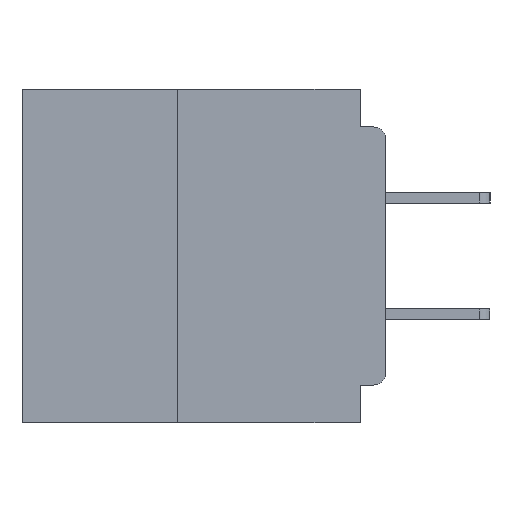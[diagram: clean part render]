
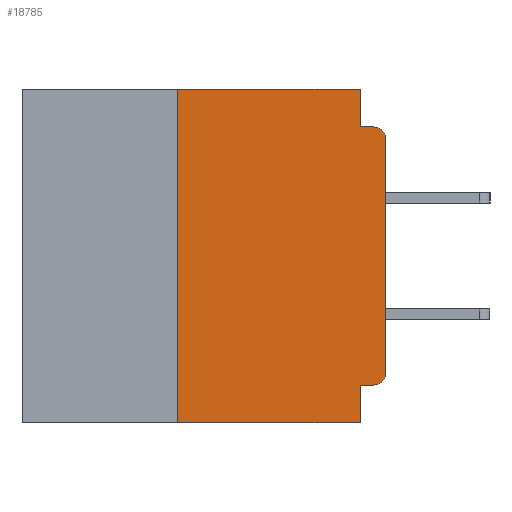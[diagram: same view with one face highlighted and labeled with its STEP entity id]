
A CAD part, left-side view. The second image highlights one B-rep face of the part: STEP entity #18785.
In plain terms, the highlighted planar face has unit normal (-1, 0, 0).
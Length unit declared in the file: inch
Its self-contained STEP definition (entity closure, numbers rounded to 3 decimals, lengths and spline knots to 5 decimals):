
#663 = CARTESIAN_POINT ( 'NONE',  ( 0., 0.015, -0.355 ) ) ;
#713 = CARTESIAN_POINT ( 'NONE',  ( 0., 0.031, -0.4 ) ) ;
#2166 = VERTEX_POINT ( 'NONE', #713 ) ;
#2674 = CARTESIAN_POINT ( 'NONE',  ( 0., 0., -0.355 ) ) ;
#2922 = VERTEX_POINT ( 'NONE', #11174 ) ;
#4207 = CARTESIAN_POINT ( 'NONE',  ( 0., 0.031, -0.045 ) ) ;
#4211 = ORIENTED_EDGE ( 'NONE', *, *, #28595, .T. ) ;
#5826 = VERTEX_POINT ( 'NONE', #27957 ) ;
#6435 = LINE ( 'NONE', #2674, #48148 ) ;
#7104 = VECTOR ( 'NONE', #25370, 39.37008 ) ;
#8493 = CARTESIAN_POINT ( 'NONE',  ( 0., 0., -0.045 ) ) ;
#8925 = AXIS2_PLACEMENT_3D ( 'NONE', #42290, #46321, #22133 ) ;
#9164 = EDGE_LOOP ( 'NONE', ( #46527, #39739, #34785, #50133, #48229, #15611, #4211, #15721, #17153, #42889 ) ) ;
#9626 = LINE ( 'NONE', #43759, #43172 ) ;
#9649 = LINE ( 'NONE', #8493, #19128 ) ;
#9907 = DIRECTION ( 'NONE',  ( 0., -1., 0. ) ) ;
#11011 = VECTOR ( 'NONE', #44878, 39.37008 ) ;
#11174 = CARTESIAN_POINT ( 'NONE',  ( 0., 0.25, 0. ) ) ;
#11696 = DIRECTION ( 'NONE',  ( -1., 0., 0. ) ) ;
#12489 = VERTEX_POINT ( 'NONE', #25854 ) ;
#12490 = CARTESIAN_POINT ( 'NONE',  ( 0., 0.25, -0.4 ) ) ;
#12646 = EDGE_CURVE ( 'NONE', #14456, #12489, #6435, .T. ) ;
#13165 = DIRECTION ( 'NONE',  ( 0., 0., -1. ) ) ;
#13948 = PLANE ( 'NONE',  #8925 ) ;
#14456 = VERTEX_POINT ( 'NONE', #663 ) ;
#15611 = ORIENTED_EDGE ( 'NONE', *, *, #50242, .F. ) ;
#15721 = ORIENTED_EDGE ( 'NONE', *, *, #23178, .F. ) ;
#16581 = VERTEX_POINT ( 'NONE', #30914 ) ;
#17153 = ORIENTED_EDGE ( 'NONE', *, *, #12646, .F. ) ;
#17453 = VERTEX_POINT ( 'NONE', #24900 ) ;
#18785 = ADVANCED_FACE ( 'NONE', ( #31189 ), #13948, .F. ) ;
#19089 = LINE ( 'NONE', #45521, #7104 ) ;
#19128 = VECTOR ( 'NONE', #28628, 39.37008 ) ;
#19195 = EDGE_CURVE ( 'NONE', #45797, #17453, #9649, .T. ) ;
#19537 = DIRECTION ( 'NONE',  ( 0., 0., -1. ) ) ;
#20698 = VERTEX_POINT ( 'NONE', #33028 ) ;
#22133 = DIRECTION ( 'NONE',  ( 0., 0., -1. ) ) ;
#22605 = CARTESIAN_POINT ( 'NONE',  ( 0., 0.015, -0.06 ) ) ;
#23178 = EDGE_CURVE ( 'NONE', #12489, #2166, #38935, .T. ) ;
#24900 = CARTESIAN_POINT ( 'NONE',  ( 0., 0.015, -0.045 ) ) ;
#25370 = DIRECTION ( 'NONE',  ( 0., 0., 1. ) ) ;
#25854 = CARTESIAN_POINT ( 'NONE',  ( 0., 0.031, -0.355 ) ) ;
#26081 = CIRCLE ( 'NONE', #33354, 0.015 ) ;
#26270 = VECTOR ( 'NONE', #9907, 39.37008 ) ;
#26529 = AXIS2_PLACEMENT_3D ( 'NONE', #35959, #11696, #40004 ) ;
#26676 = DIRECTION ( 'NONE',  ( 0., 0., -1. ) ) ;
#27008 = EDGE_CURVE ( 'NONE', #2922, #5826, #46505, .T. ) ;
#27957 = CARTESIAN_POINT ( 'NONE',  ( 0., 0.031, 0. ) ) ;
#28595 = EDGE_CURVE ( 'NONE', #20698, #2166, #45693, .T. ) ;
#28628 = DIRECTION ( 'NONE',  ( 0., -1., 0. ) ) ;
#30914 = CARTESIAN_POINT ( 'NONE',  ( 0., 0., -0.34 ) ) ;
#31189 = FACE_OUTER_BOUND ( 'NONE', #9164, .T. ) ;
#33028 = CARTESIAN_POINT ( 'NONE',  ( 0., 0.25, -0.4 ) ) ;
#33335 = EDGE_CURVE ( 'NONE', #14456, #16581, #41442, .T. ) ;
#33354 = AXIS2_PLACEMENT_3D ( 'NONE', #22605, #50775, #26676 ) ;
#33555 = CARTESIAN_POINT ( 'NONE',  ( 0., 0.031, -0.4 ) ) ;
#34110 = CARTESIAN_POINT ( 'NONE',  ( 0., 0.437, 0. ) ) ;
#34453 = EDGE_CURVE ( 'NONE', #35327, #17453, #26081, .T. ) ;
#34785 = ORIENTED_EDGE ( 'NONE', *, *, #19195, .F. ) ;
#34903 = EDGE_CURVE ( 'NONE', #16581, #35327, #19089, .T. ) ;
#34961 = VECTOR ( 'NONE', #44053, 39.37008 ) ;
#35327 = VERTEX_POINT ( 'NONE', #40776 ) ;
#35959 = CARTESIAN_POINT ( 'NONE',  ( 0., 0.015, -0.34 ) ) ;
#38935 = LINE ( 'NONE', #33555, #48385 ) ;
#39739 = ORIENTED_EDGE ( 'NONE', *, *, #34453, .T. ) ;
#39983 = CARTESIAN_POINT ( 'NONE',  ( 0., 0.437, -0.4 ) ) ;
#40004 = DIRECTION ( 'NONE',  ( 0., 0., -1. ) ) ;
#40776 = CARTESIAN_POINT ( 'NONE',  ( 0., 0., -0.06 ) ) ;
#41442 = CIRCLE ( 'NONE', #26529, 0.015 ) ;
#42034 = LINE ( 'NONE', #12490, #11011 ) ;
#42290 = CARTESIAN_POINT ( 'NONE',  ( 0., 0.437, 0. ) ) ;
#42415 = EDGE_CURVE ( 'NONE', #5826, #45797, #9626, .T. ) ;
#42889 = ORIENTED_EDGE ( 'NONE', *, *, #33335, .T. ) ;
#43172 = VECTOR ( 'NONE', #19537, 39.37008 ) ;
#43759 = CARTESIAN_POINT ( 'NONE',  ( 0., 0.031, 0. ) ) ;
#44053 = DIRECTION ( 'NONE',  ( 0., -1., 0. ) ) ;
#44878 = DIRECTION ( 'NONE',  ( 0., 0., 1. ) ) ;
#45521 = CARTESIAN_POINT ( 'NONE',  ( 0., 0., 0. ) ) ;
#45693 = LINE ( 'NONE', #39983, #34961 ) ;
#45797 = VERTEX_POINT ( 'NONE', #4207 ) ;
#46321 = DIRECTION ( 'NONE',  ( 1., 0., 0. ) ) ;
#46505 = LINE ( 'NONE', #34110, #26270 ) ;
#46527 = ORIENTED_EDGE ( 'NONE', *, *, #34903, .T. ) ;
#48148 = VECTOR ( 'NONE', #51017, 39.37008 ) ;
#48229 = ORIENTED_EDGE ( 'NONE', *, *, #27008, .F. ) ;
#48385 = VECTOR ( 'NONE', #13165, 39.37008 ) ;
#50133 = ORIENTED_EDGE ( 'NONE', *, *, #42415, .F. ) ;
#50242 = EDGE_CURVE ( 'NONE', #20698, #2922, #42034, .T. ) ;
#50775 = DIRECTION ( 'NONE',  ( -1., 0., 0. ) ) ;
#51017 = DIRECTION ( 'NONE',  ( 0., 1., 0. ) ) ;
